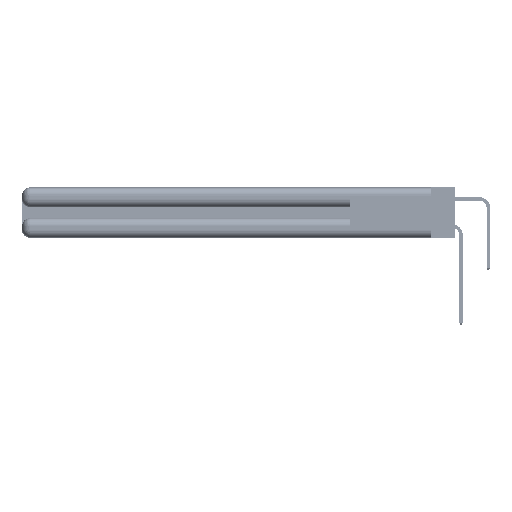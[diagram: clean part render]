
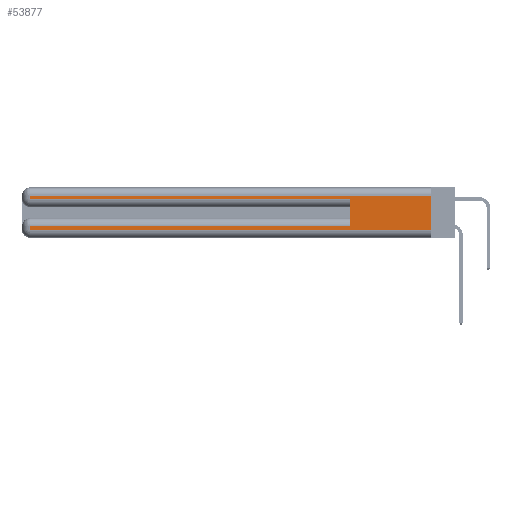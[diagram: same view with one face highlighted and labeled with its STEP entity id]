
A CAD part, left-side view. The second image highlights one B-rep face of the part: STEP entity #53877.
In plain terms, the highlighted planar face has unit normal (-1, 0, 0).
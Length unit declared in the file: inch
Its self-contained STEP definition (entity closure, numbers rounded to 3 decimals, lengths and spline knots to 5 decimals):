
#1532 = DIRECTION ( 'NONE',  ( 0., 1., 0. ) ) ;
#2345 = CARTESIAN_POINT ( 'NONE',  ( 0., 0.6, 0.285 ) ) ;
#3156 = LINE ( 'NONE', #53428, #43803 ) ;
#7156 = LINE ( 'NONE', #30482, #50280 ) ;
#7729 = VERTEX_POINT ( 'NONE', #45759 ) ;
#8641 = VECTOR ( 'NONE', #50976, 39.37008 ) ;
#8763 = LINE ( 'NONE', #32122, #29890 ) ;
#10917 = ORIENTED_EDGE ( 'NONE', *, *, #42605, .F. ) ;
#11887 = PLANE ( 'NONE',  #26790 ) ;
#13452 = DIRECTION ( 'NONE',  ( 0., 0., -1. ) ) ;
#14938 = VERTEX_POINT ( 'NONE', #2345 ) ;
#15343 = DIRECTION ( 'NONE',  ( 0., 1., 0. ) ) ;
#15379 = EDGE_CURVE ( 'NONE', #23242, #32314, #49582, .T. ) ;
#17063 = VECTOR ( 'NONE', #54197, 39.37008 ) ;
#17816 = DIRECTION ( 'NONE',  ( 0., 0., -1. ) ) ;
#18884 = EDGE_CURVE ( 'NONE', #37348, #7729, #47909, .T. ) ;
#18906 = ORIENTED_EDGE ( 'NONE', *, *, #19302, .T. ) ;
#19302 = EDGE_CURVE ( 'NONE', #32314, #50265, #51740, .T. ) ;
#19795 = CARTESIAN_POINT ( 'NONE',  ( 0., 0., 0.31 ) ) ;
#20024 = LINE ( 'NONE', #31096, #39592 ) ;
#20426 = DIRECTION ( 'NONE',  ( 0., 0., -1. ) ) ;
#21029 = CARTESIAN_POINT ( 'NONE',  ( 0., 2.94, 0.37 ) ) ;
#23242 = VERTEX_POINT ( 'NONE', #44826 ) ;
#23398 = CARTESIAN_POINT ( 'NONE',  ( 0., 2.94, 0.06 ) ) ;
#23438 = VERTEX_POINT ( 'NONE', #25443 ) ;
#25443 = CARTESIAN_POINT ( 'NONE',  ( 0., 2.94, 0.285 ) ) ;
#25871 = VECTOR ( 'NONE', #15343, 39.37008 ) ;
#26168 = CARTESIAN_POINT ( 'NONE',  ( 0., 0., 0.06 ) ) ;
#26790 = AXIS2_PLACEMENT_3D ( 'NONE', #41141, #45298, #20426 ) ;
#28277 = LINE ( 'NONE', #21029, #17063 ) ;
#29086 = CARTESIAN_POINT ( 'NONE',  ( 0., 0., 0.06 ) ) ;
#29890 = VECTOR ( 'NONE', #40440, 39.37008 ) ;
#30135 = EDGE_CURVE ( 'NONE', #37348, #50265, #7156, .T. ) ;
#30482 = CARTESIAN_POINT ( 'NONE',  ( 0., 0., 0.37 ) ) ;
#31096 = CARTESIAN_POINT ( 'NONE',  ( 0., 0., 0.085 ) ) ;
#31959 = ORIENTED_EDGE ( 'NONE', *, *, #50537, .T. ) ;
#32122 = CARTESIAN_POINT ( 'NONE',  ( 0., 0., 0.285 ) ) ;
#32314 = VERTEX_POINT ( 'NONE', #23398 ) ;
#34036 = FACE_OUTER_BOUND ( 'NONE', #50190, .T. ) ;
#35875 = ORIENTED_EDGE ( 'NONE', *, *, #49897, .T. ) ;
#37321 = VECTOR ( 'NONE', #13452, 39.37008 ) ;
#37348 = VERTEX_POINT ( 'NONE', #19795 ) ;
#39096 = ORIENTED_EDGE ( 'NONE', *, *, #18884, .T. ) ;
#39592 = VECTOR ( 'NONE', #1532, 39.37008 ) ;
#40375 = ORIENTED_EDGE ( 'NONE', *, *, #53300, .T. ) ;
#40440 = DIRECTION ( 'NONE',  ( 0., -1., 0. ) ) ;
#41141 = CARTESIAN_POINT ( 'NONE',  ( 0., 0., 0.37 ) ) ;
#42605 = EDGE_CURVE ( 'NONE', #48585, #14938, #3156, .T. ) ;
#43803 = VECTOR ( 'NONE', #45474, 39.37008 ) ;
#44826 = CARTESIAN_POINT ( 'NONE',  ( 0., 2.94, 0.085 ) ) ;
#45298 = DIRECTION ( 'NONE',  ( 1., 0., 0. ) ) ;
#45474 = DIRECTION ( 'NONE',  ( 0., 0., 1. ) ) ;
#45759 = CARTESIAN_POINT ( 'NONE',  ( 0., 2.94, 0.31 ) ) ;
#46816 = CARTESIAN_POINT ( 'NONE',  ( 0., 2.94, 0.37 ) ) ;
#47909 = LINE ( 'NONE', #52638, #25871 ) ;
#48163 = ORIENTED_EDGE ( 'NONE', *, *, #15379, .T. ) ;
#48585 = VERTEX_POINT ( 'NONE', #51779 ) ;
#48782 = ORIENTED_EDGE ( 'NONE', *, *, #30135, .F. ) ;
#49582 = LINE ( 'NONE', #46816, #37321 ) ;
#49897 = EDGE_CURVE ( 'NONE', #48585, #23242, #20024, .T. ) ;
#50190 = EDGE_LOOP ( 'NONE', ( #48782, #39096, #40375, #31959, #10917, #35875, #48163, #18906 ) ) ;
#50265 = VERTEX_POINT ( 'NONE', #29086 ) ;
#50280 = VECTOR ( 'NONE', #17816, 39.37008 ) ;
#50537 = EDGE_CURVE ( 'NONE', #23438, #14938, #8763, .T. ) ;
#50976 = DIRECTION ( 'NONE',  ( 0., -1., 0. ) ) ;
#51740 = LINE ( 'NONE', #26168, #8641 ) ;
#51779 = CARTESIAN_POINT ( 'NONE',  ( 0., 0.6, 0.085 ) ) ;
#52638 = CARTESIAN_POINT ( 'NONE',  ( 0., 0., 0.31 ) ) ;
#53300 = EDGE_CURVE ( 'NONE', #7729, #23438, #28277, .T. ) ;
#53428 = CARTESIAN_POINT ( 'NONE',  ( 0., 0.6, 0.145 ) ) ;
#53877 = ADVANCED_FACE ( 'NONE', ( #34036 ), #11887, .F. ) ;
#54197 = DIRECTION ( 'NONE',  ( 0., 0., -1. ) ) ;
